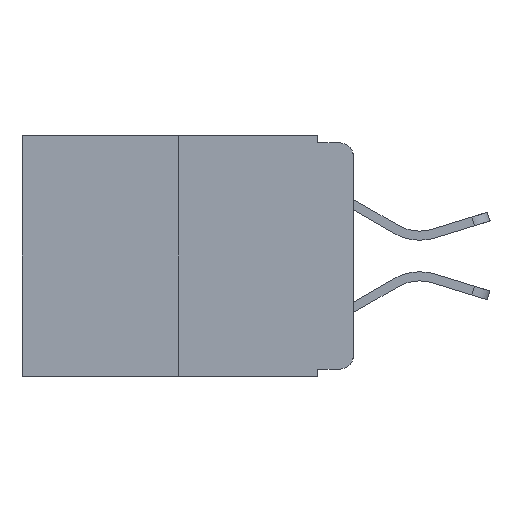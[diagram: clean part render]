
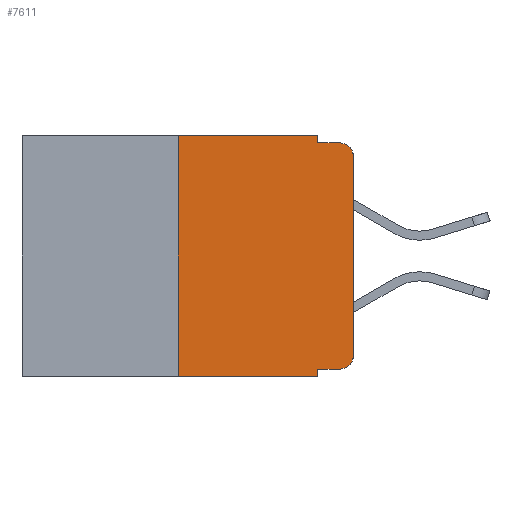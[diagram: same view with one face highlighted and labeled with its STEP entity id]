
A CAD part, left-side view. The second image highlights one B-rep face of the part: STEP entity #7611.
In plain terms, the highlighted planar face has unit normal (-1, 0, 0).
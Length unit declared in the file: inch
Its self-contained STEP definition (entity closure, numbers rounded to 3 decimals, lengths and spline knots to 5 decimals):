
#429 = CARTESIAN_POINT ( 'NONE',  ( 0., 0.473, 0. ) ) ;
#541 = DIRECTION ( 'NONE',  ( 1., 0., 0. ) ) ;
#598 = CARTESIAN_POINT ( 'NONE',  ( 0., 0.02, -0.333 ) ) ;
#605 = VECTOR ( 'NONE', #9368, 39.37008 ) ;
#660 = DIRECTION ( 'NONE',  ( 0., 0., -1. ) ) ;
#818 = ORIENTED_EDGE ( 'NONE', *, *, #2142, .T. ) ;
#1044 = LINE ( 'NONE', #4914, #9555 ) ;
#1052 = ORIENTED_EDGE ( 'NONE', *, *, #6600, .T. ) ;
#1120 = ORIENTED_EDGE ( 'NONE', *, *, #2902, .T. ) ;
#1156 = VERTEX_POINT ( 'NONE', #1926 ) ;
#1198 = CARTESIAN_POINT ( 'NONE',  ( 0., 0.25, 0. ) ) ;
#1424 = VERTEX_POINT ( 'NONE', #6569 ) ;
#1926 = CARTESIAN_POINT ( 'NONE',  ( 0., 0.25, -0.343 ) ) ;
#2142 = EDGE_CURVE ( 'NONE', #12383, #5305, #3748, .T. ) ;
#2323 = ORIENTED_EDGE ( 'NONE', *, *, #5141, .F. ) ;
#2643 = VECTOR ( 'NONE', #6550, 39.37008 ) ;
#2681 = CARTESIAN_POINT ( 'NONE',  ( 0., 0.473, 0. ) ) ;
#2727 = ORIENTED_EDGE ( 'NONE', *, *, #5852, .F. ) ;
#2902 = EDGE_CURVE ( 'NONE', #3648, #12383, #13777, .T. ) ;
#2923 = FACE_OUTER_BOUND ( 'NONE', #10030, .T. ) ;
#3078 = DIRECTION ( 'NONE',  ( -1., 0., 0. ) ) ;
#3154 = LINE ( 'NONE', #7339, #5744 ) ;
#3601 = ORIENTED_EDGE ( 'NONE', *, *, #4378, .F. ) ;
#3633 = EDGE_CURVE ( 'NONE', #3648, #1424, #1044, .T. ) ;
#3648 = VERTEX_POINT ( 'NONE', #11364 ) ;
#3655 = EDGE_CURVE ( 'NONE', #10454, #5692, #3718, .T. ) ;
#3718 = LINE ( 'NONE', #2681, #605 ) ;
#3748 = CIRCLE ( 'NONE', #4559, 0.02 ) ;
#4378 = EDGE_CURVE ( 'NONE', #1156, #10454, #13280, .T. ) ;
#4559 = AXIS2_PLACEMENT_3D ( 'NONE', #11621, #3078, #660 ) ;
#4595 = ORIENTED_EDGE ( 'NONE', *, *, #3655, .F. ) ;
#4657 = DIRECTION ( 'NONE',  ( 0., -1., 0. ) ) ;
#4661 = VERTEX_POINT ( 'NONE', #12141 ) ;
#4914 = CARTESIAN_POINT ( 'NONE',  ( 0., 0.051, 0. ) ) ;
#5141 = EDGE_CURVE ( 'NONE', #5692, #4661, #5576, .T. ) ;
#5305 = VERTEX_POINT ( 'NONE', #9734 ) ;
#5348 = CARTESIAN_POINT ( 'NONE',  ( 0., 0.02, -0.01 ) ) ;
#5576 = LINE ( 'NONE', #8649, #2643 ) ;
#5692 = VERTEX_POINT ( 'NONE', #13721 ) ;
#5744 = VECTOR ( 'NONE', #7203, 39.37008 ) ;
#5852 = EDGE_CURVE ( 'NONE', #4661, #13255, #3154, .T. ) ;
#5922 = ORIENTED_EDGE ( 'NONE', *, *, #7354, .T. ) ;
#6032 = CARTESIAN_POINT ( 'NONE',  ( 0., 0.051, -0.333 ) ) ;
#6124 = CARTESIAN_POINT ( 'NONE',  ( 0., 0.02, -0.03 ) ) ;
#6317 = LINE ( 'NONE', #13053, #8898 ) ;
#6371 = ORIENTED_EDGE ( 'NONE', *, *, #3633, .F. ) ;
#6550 = DIRECTION ( 'NONE',  ( 0., 0., -1. ) ) ;
#6569 = CARTESIAN_POINT ( 'NONE',  ( 0., 0.051, -0.343 ) ) ;
#6586 = DIRECTION ( 'NONE',  ( 0., 0., 1. ) ) ;
#6600 = EDGE_CURVE ( 'NONE', #9018, #13255, #9330, .T. ) ;
#7018 = AXIS2_PLACEMENT_3D ( 'NONE', #429, #541, #8473 ) ;
#7200 = ORIENTED_EDGE ( 'NONE', *, *, #11991, .T. ) ;
#7203 = DIRECTION ( 'NONE',  ( 0., -1., 0. ) ) ;
#7250 = DIRECTION ( 'NONE',  ( 0., 0., -1. ) ) ;
#7339 = CARTESIAN_POINT ( 'NONE',  ( 0., 0.051, -0.01 ) ) ;
#7354 = EDGE_CURVE ( 'NONE', #5305, #9018, #7444, .T. ) ;
#7444 = LINE ( 'NONE', #12796, #12584 ) ;
#7611 = ADVANCED_FACE ( 'NONE', ( #2923 ), #12506, .F. ) ;
#8224 = VECTOR ( 'NONE', #11076, 39.37008 ) ;
#8428 = VECTOR ( 'NONE', #13043, 39.37008 ) ;
#8473 = DIRECTION ( 'NONE',  ( 0., 0., -1. ) ) ;
#8649 = CARTESIAN_POINT ( 'NONE',  ( 0., 0.051, 0. ) ) ;
#8898 = VECTOR ( 'NONE', #4657, 39.37008 ) ;
#9018 = VERTEX_POINT ( 'NONE', #12324 ) ;
#9272 = DIRECTION ( 'NONE',  ( 0., 0., -1. ) ) ;
#9330 = CIRCLE ( 'NONE', #12084, 0.02 ) ;
#9368 = DIRECTION ( 'NONE',  ( 0., -1., 0. ) ) ;
#9555 = VECTOR ( 'NONE', #9272, 39.37008 ) ;
#9734 = CARTESIAN_POINT ( 'NONE',  ( 0., 0., -0.313 ) ) ;
#10030 = EDGE_LOOP ( 'NONE', ( #5922, #1052, #2727, #2323, #4595, #3601, #7200, #6371, #1120, #818 ) ) ;
#10454 = VERTEX_POINT ( 'NONE', #12944 ) ;
#11076 = DIRECTION ( 'NONE',  ( 0., 0., 1. ) ) ;
#11364 = CARTESIAN_POINT ( 'NONE',  ( 0., 0.051, -0.333 ) ) ;
#11621 = CARTESIAN_POINT ( 'NONE',  ( 0., 0.02, -0.313 ) ) ;
#11991 = EDGE_CURVE ( 'NONE', #1156, #1424, #6317, .T. ) ;
#12084 = AXIS2_PLACEMENT_3D ( 'NONE', #6124, #13388, #7250 ) ;
#12141 = CARTESIAN_POINT ( 'NONE',  ( 0., 0.051, -0.01 ) ) ;
#12324 = CARTESIAN_POINT ( 'NONE',  ( 0., 0., -0.03 ) ) ;
#12383 = VERTEX_POINT ( 'NONE', #598 ) ;
#12506 = PLANE ( 'NONE',  #7018 ) ;
#12584 = VECTOR ( 'NONE', #6586, 39.37008 ) ;
#12796 = CARTESIAN_POINT ( 'NONE',  ( 0., 0., 0. ) ) ;
#12944 = CARTESIAN_POINT ( 'NONE',  ( 0., 0.25, 0. ) ) ;
#13043 = DIRECTION ( 'NONE',  ( 0., -1., 0. ) ) ;
#13053 = CARTESIAN_POINT ( 'NONE',  ( 0., 0.473, -0.343 ) ) ;
#13255 = VERTEX_POINT ( 'NONE', #5348 ) ;
#13280 = LINE ( 'NONE', #1198, #8224 ) ;
#13388 = DIRECTION ( 'NONE',  ( -1., 0., 0. ) ) ;
#13721 = CARTESIAN_POINT ( 'NONE',  ( 0., 0.051, 0. ) ) ;
#13777 = LINE ( 'NONE', #6032, #8428 ) ;
